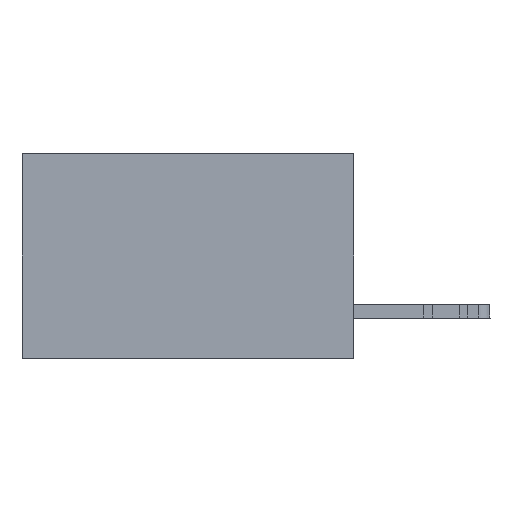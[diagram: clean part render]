
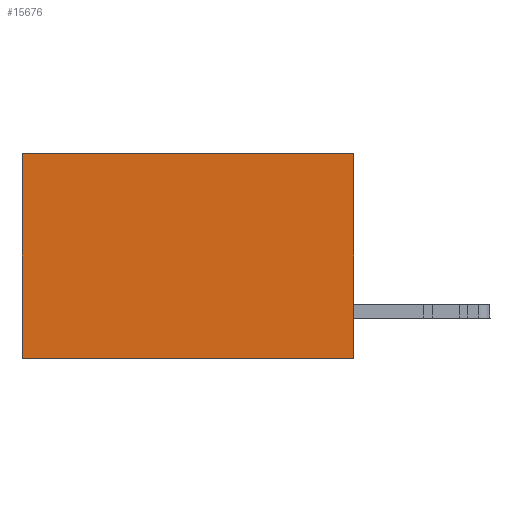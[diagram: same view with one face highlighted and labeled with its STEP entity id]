
A CAD part, left-side view. The second image highlights one B-rep face of the part: STEP entity #15676.
In plain terms, the highlighted planar face has unit normal (-1, 0, 0).
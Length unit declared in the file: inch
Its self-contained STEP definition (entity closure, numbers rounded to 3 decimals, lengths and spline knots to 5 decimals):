
#483 = EDGE_CURVE ( 'NONE', #46925, #31545, #6520, .T. ) ;
#2196 = ORIENTED_EDGE ( 'NONE', *, *, #43268, .T. ) ;
#4687 = LINE ( 'NONE', #40462, #5835 ) ;
#4696 = VERTEX_POINT ( 'NONE', #21152 ) ;
#4789 = CARTESIAN_POINT ( 'NONE',  ( 0.2875, 0.6, 0. ) ) ;
#5835 = VECTOR ( 'NONE', #14620, 39.37008 ) ;
#6520 = LINE ( 'NONE', #4789, #33955 ) ;
#7815 = PLANE ( 'NONE',  #34244 ) ;
#7937 = CARTESIAN_POINT ( 'NONE',  ( 0.2875, 0., -0.37 ) ) ;
#8448 = DIRECTION ( 'NONE',  ( 0., 0., -1. ) ) ;
#9926 = EDGE_LOOP ( 'NONE', ( #11975, #25828, #14850, #2196 ) ) ;
#11975 = ORIENTED_EDGE ( 'NONE', *, *, #483, .T. ) ;
#14187 = EDGE_CURVE ( 'NONE', #4696, #33375, #4687, .T. ) ;
#14620 = DIRECTION ( 'NONE',  ( 0., 0., -1. ) ) ;
#14822 = CARTESIAN_POINT ( 'NONE',  ( 0.2875, 0.6, -0.37 ) ) ;
#14850 = ORIENTED_EDGE ( 'NONE', *, *, #14187, .F. ) ;
#15047 = DIRECTION ( 'NONE',  ( 0., 1., 0. ) ) ;
#15676 = ADVANCED_FACE ( 'NONE', ( #18232 ), #7815, .F. ) ;
#18232 = FACE_OUTER_BOUND ( 'NONE', #9926, .T. ) ;
#21152 = CARTESIAN_POINT ( 'NONE',  ( 0.2875, 0., 0. ) ) ;
#22313 = CARTESIAN_POINT ( 'NONE',  ( 0.2875, 0., 0. ) ) ;
#25828 = ORIENTED_EDGE ( 'NONE', *, *, #29578, .F. ) ;
#29578 = EDGE_CURVE ( 'NONE', #33375, #31545, #41878, .T. ) ;
#29847 = DIRECTION ( 'NONE',  ( 0., 1., 0. ) ) ;
#30939 = LINE ( 'NONE', #36755, #34357 ) ;
#31545 = VERTEX_POINT ( 'NONE', #14822 ) ;
#32005 = CARTESIAN_POINT ( 'NONE',  ( 0.2875, 0.6, 0. ) ) ;
#33375 = VERTEX_POINT ( 'NONE', #34609 ) ;
#33859 = VECTOR ( 'NONE', #29847, 39.37008 ) ;
#33955 = VECTOR ( 'NONE', #8448, 39.37008 ) ;
#34244 = AXIS2_PLACEMENT_3D ( 'NONE', #22313, #37014, #44526 ) ;
#34357 = VECTOR ( 'NONE', #15047, 39.37008 ) ;
#34609 = CARTESIAN_POINT ( 'NONE',  ( 0.2875, 0., -0.37 ) ) ;
#36755 = CARTESIAN_POINT ( 'NONE',  ( 0.2875, 0., 0. ) ) ;
#37014 = DIRECTION ( 'NONE',  ( 1., 0., 0. ) ) ;
#40462 = CARTESIAN_POINT ( 'NONE',  ( 0.2875, 0., 0. ) ) ;
#41878 = LINE ( 'NONE', #7937, #33859 ) ;
#43268 = EDGE_CURVE ( 'NONE', #4696, #46925, #30939, .T. ) ;
#44526 = DIRECTION ( 'NONE',  ( 0., 0., -1. ) ) ;
#46925 = VERTEX_POINT ( 'NONE', #32005 ) ;
